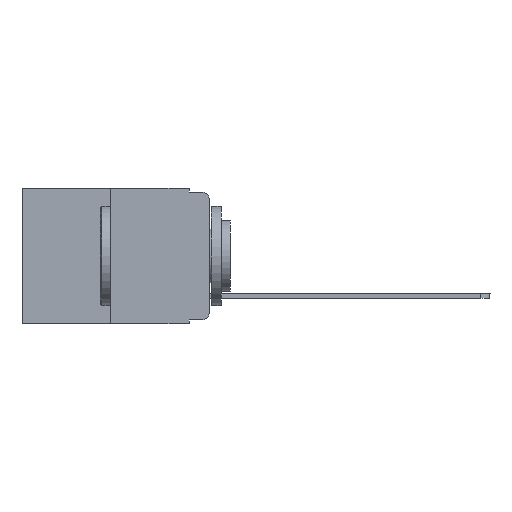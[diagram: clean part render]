
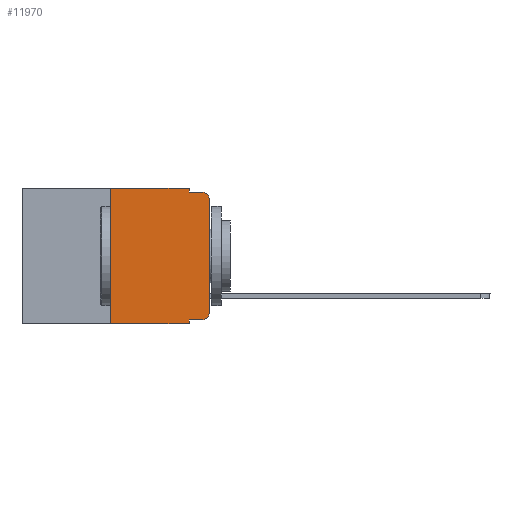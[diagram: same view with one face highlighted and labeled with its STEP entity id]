
A CAD part, left-side view. The second image highlights one B-rep face of the part: STEP entity #11970.
In plain terms, the highlighted planar face has unit normal (-1, 0, 0).
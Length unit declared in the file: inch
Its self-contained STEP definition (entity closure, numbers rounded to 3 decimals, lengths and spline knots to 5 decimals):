
#198 = CIRCLE ( 'NONE', #10789, 0.02 ) ;
#292 = EDGE_LOOP ( 'NONE', ( #4827, #2773, #5858, #7599, #11472, #8282, #11973, #1126, #9190, #11905 ) ) ;
#298 = CARTESIAN_POINT ( 'NONE',  ( 0., 0.473, -0.343 ) ) ;
#349 = CARTESIAN_POINT ( 'NONE',  ( 0., 0.25, -0.343 ) ) ;
#738 = CARTESIAN_POINT ( 'NONE',  ( 0., 0.02, -0.333 ) ) ;
#879 = VECTOR ( 'NONE', #5406, 39.37008 ) ;
#992 = FACE_OUTER_BOUND ( 'NONE', #292, .T. ) ;
#1126 = ORIENTED_EDGE ( 'NONE', *, *, #4000, .F. ) ;
#1228 = LINE ( 'NONE', #4236, #6453 ) ;
#1486 = DIRECTION ( 'NONE',  ( 0., -1., 0. ) ) ;
#1525 = EDGE_CURVE ( 'NONE', #5626, #4326, #9640, .T. ) ;
#1549 = DIRECTION ( 'NONE',  ( 0., 0., -1. ) ) ;
#1772 = CARTESIAN_POINT ( 'NONE',  ( 0., 0.02, -0.01 ) ) ;
#1840 = LINE ( 'NONE', #5749, #6718 ) ;
#1992 = PLANE ( 'NONE',  #6631 ) ;
#2773 = ORIENTED_EDGE ( 'NONE', *, *, #3183, .T. ) ;
#3183 = EDGE_CURVE ( 'NONE', #6879, #10955, #198, .T. ) ;
#3437 = LINE ( 'NONE', #298, #8593 ) ;
#3528 = DIRECTION ( 'NONE',  ( 0., 0., -1. ) ) ;
#3816 = DIRECTION ( 'NONE',  ( 1., 0., 0. ) ) ;
#4000 = EDGE_CURVE ( 'NONE', #8976, #6531, #4372, .T. ) ;
#4071 = EDGE_CURVE ( 'NONE', #4326, #10955, #1840, .T. ) ;
#4105 = DIRECTION ( 'NONE',  ( 0., -1., 0. ) ) ;
#4229 = VECTOR ( 'NONE', #3528, 39.37008 ) ;
#4236 = CARTESIAN_POINT ( 'NONE',  ( 0., 0.051, -0.333 ) ) ;
#4326 = VERTEX_POINT ( 'NONE', #7346 ) ;
#4336 = CARTESIAN_POINT ( 'NONE',  ( 0., 0.051, -0.333 ) ) ;
#4372 = LINE ( 'NONE', #8394, #879 ) ;
#4461 = VERTEX_POINT ( 'NONE', #12693 ) ;
#4827 = ORIENTED_EDGE ( 'NONE', *, *, #10205, .T. ) ;
#5384 = LINE ( 'NONE', #9339, #11260 ) ;
#5406 = DIRECTION ( 'NONE',  ( 0., 0., -1. ) ) ;
#5626 = VERTEX_POINT ( 'NONE', #9163 ) ;
#5749 = CARTESIAN_POINT ( 'NONE',  ( 0., 0.051, -0.01 ) ) ;
#5858 = ORIENTED_EDGE ( 'NONE', *, *, #4071, .F. ) ;
#6405 = VERTEX_POINT ( 'NONE', #6517 ) ;
#6453 = VECTOR ( 'NONE', #4105, 39.37008 ) ;
#6517 = CARTESIAN_POINT ( 'NONE',  ( 0., 0.25, 0. ) ) ;
#6531 = VERTEX_POINT ( 'NONE', #12653 ) ;
#6554 = CARTESIAN_POINT ( 'NONE',  ( 0., 0., 0. ) ) ;
#6628 = EDGE_CURVE ( 'NONE', #9157, #4461, #8530, .T. ) ;
#6631 = AXIS2_PLACEMENT_3D ( 'NONE', #10020, #3816, #9895 ) ;
#6718 = VECTOR ( 'NONE', #9695, 39.37008 ) ;
#6749 = EDGE_CURVE ( 'NONE', #8976, #9157, #1228, .T. ) ;
#6879 = VERTEX_POINT ( 'NONE', #11352 ) ;
#7158 = DIRECTION ( 'NONE',  ( -1., 0., 0. ) ) ;
#7319 = VERTEX_POINT ( 'NONE', #349 ) ;
#7346 = CARTESIAN_POINT ( 'NONE',  ( 0., 0.051, -0.01 ) ) ;
#7599 = ORIENTED_EDGE ( 'NONE', *, *, #1525, .F. ) ;
#7873 = VECTOR ( 'NONE', #8428, 39.37008 ) ;
#8282 = ORIENTED_EDGE ( 'NONE', *, *, #8654, .F. ) ;
#8394 = CARTESIAN_POINT ( 'NONE',  ( 0., 0.051, 0. ) ) ;
#8428 = DIRECTION ( 'NONE',  ( 0., 0., 1. ) ) ;
#8463 = CARTESIAN_POINT ( 'NONE',  ( 0., 0.051, 0. ) ) ;
#8524 = VECTOR ( 'NONE', #9856, 39.37008 ) ;
#8530 = CIRCLE ( 'NONE', #10994, 0.02 ) ;
#8593 = VECTOR ( 'NONE', #1486, 39.37008 ) ;
#8654 = EDGE_CURVE ( 'NONE', #7319, #6405, #5384, .T. ) ;
#8655 = EDGE_CURVE ( 'NONE', #7319, #6531, #3437, .T. ) ;
#8976 = VERTEX_POINT ( 'NONE', #4336 ) ;
#9157 = VERTEX_POINT ( 'NONE', #738 ) ;
#9163 = CARTESIAN_POINT ( 'NONE',  ( 0., 0.051, 0. ) ) ;
#9190 = ORIENTED_EDGE ( 'NONE', *, *, #6749, .T. ) ;
#9339 = CARTESIAN_POINT ( 'NONE',  ( 0., 0.25, 0. ) ) ;
#9640 = LINE ( 'NONE', #8463, #4229 ) ;
#9695 = DIRECTION ( 'NONE',  ( 0., -1., 0. ) ) ;
#9728 = LINE ( 'NONE', #6554, #7873 ) ;
#9800 = CARTESIAN_POINT ( 'NONE',  ( 0., 0.473, 0. ) ) ;
#9856 = DIRECTION ( 'NONE',  ( 0., -1., 0. ) ) ;
#9895 = DIRECTION ( 'NONE',  ( 0., 0., -1. ) ) ;
#10020 = CARTESIAN_POINT ( 'NONE',  ( 0., 0.473, 0. ) ) ;
#10205 = EDGE_CURVE ( 'NONE', #4461, #6879, #9728, .T. ) ;
#10430 = CARTESIAN_POINT ( 'NONE',  ( 0., 0.02, -0.03 ) ) ;
#10495 = DIRECTION ( 'NONE',  ( -1., 0., 0. ) ) ;
#10789 = AXIS2_PLACEMENT_3D ( 'NONE', #10430, #10495, #1549 ) ;
#10817 = LINE ( 'NONE', #9800, #8524 ) ;
#10955 = VERTEX_POINT ( 'NONE', #1772 ) ;
#10994 = AXIS2_PLACEMENT_3D ( 'NONE', #11938, #7158, #12835 ) ;
#11260 = VECTOR ( 'NONE', #11484, 39.37008 ) ;
#11352 = CARTESIAN_POINT ( 'NONE',  ( 0., 0., -0.03 ) ) ;
#11465 = EDGE_CURVE ( 'NONE', #6405, #5626, #10817, .T. ) ;
#11472 = ORIENTED_EDGE ( 'NONE', *, *, #11465, .F. ) ;
#11484 = DIRECTION ( 'NONE',  ( 0., 0., 1. ) ) ;
#11905 = ORIENTED_EDGE ( 'NONE', *, *, #6628, .T. ) ;
#11938 = CARTESIAN_POINT ( 'NONE',  ( 0., 0.02, -0.313 ) ) ;
#11970 = ADVANCED_FACE ( 'NONE', ( #992 ), #1992, .F. ) ;
#11973 = ORIENTED_EDGE ( 'NONE', *, *, #8655, .T. ) ;
#12653 = CARTESIAN_POINT ( 'NONE',  ( 0., 0.051, -0.343 ) ) ;
#12693 = CARTESIAN_POINT ( 'NONE',  ( 0., 0., -0.313 ) ) ;
#12835 = DIRECTION ( 'NONE',  ( 0., 0., -1. ) ) ;
